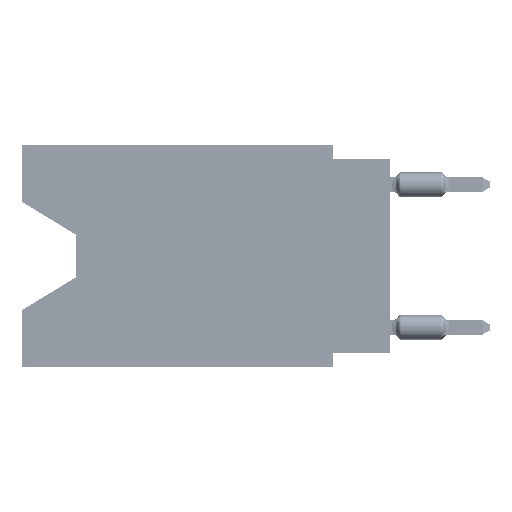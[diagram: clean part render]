
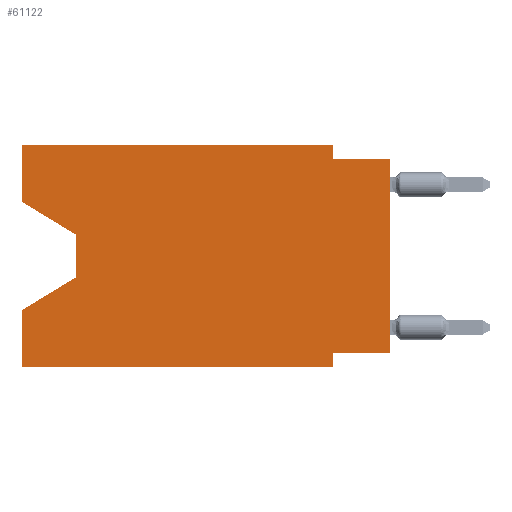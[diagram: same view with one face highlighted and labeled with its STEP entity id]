
A CAD part, left-side view. The second image highlights one B-rep face of the part: STEP entity #61122.
In plain terms, the highlighted planar face has unit normal (-1, 0, 0).
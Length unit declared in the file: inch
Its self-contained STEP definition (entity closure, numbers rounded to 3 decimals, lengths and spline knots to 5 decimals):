
#2537 = EDGE_CURVE ( 'NONE', #41093, #14408, #57321, .T. ) ;
#3447 = EDGE_CURVE ( 'NONE', #55523, #82856, #81582, .T. ) ;
#7333 = ORIENTED_EDGE ( 'NONE', *, *, #63352, .T. ) ;
#8755 = CARTESIAN_POINT ( 'NONE',  ( 0., 0.645, 0. ) ) ;
#10190 = CARTESIAN_POINT ( 'NONE',  ( 0., 0.55, -0.158 ) ) ;
#10412 = ORIENTED_EDGE ( 'NONE', *, *, #85888, .T. ) ;
#11463 = VECTOR ( 'NONE', #12196, 39.37008 ) ;
#11960 = VECTOR ( 'NONE', #19032, 39.37008 ) ;
#12196 = DIRECTION ( 'NONE',  ( 0., -1., 0. ) ) ;
#12523 = PLANE ( 'NONE',  #64655 ) ;
#13416 = EDGE_CURVE ( 'NONE', #74744, #78034, #83284, .T. ) ;
#14408 = VERTEX_POINT ( 'NONE', #86956 ) ;
#14609 = LINE ( 'NONE', #68600, #82250 ) ;
#16934 = CARTESIAN_POINT ( 'NONE',  ( 0., 0.645, 0. ) ) ;
#17168 = ORIENTED_EDGE ( 'NONE', *, *, #3447, .T. ) ;
#19032 = DIRECTION ( 'NONE',  ( 0., -1., 0. ) ) ;
#20188 = EDGE_CURVE ( 'NONE', #36233, #23892, #87376, .T. ) ;
#20350 = ORIENTED_EDGE ( 'NONE', *, *, #71336, .F. ) ;
#20557 = ORIENTED_EDGE ( 'NONE', *, *, #60749, .F. ) ;
#21324 = EDGE_CURVE ( 'NONE', #74744, #24150, #63270, .T. ) ;
#22007 = DIRECTION ( 'NONE',  ( 0., 1., 0. ) ) ;
#22513 = CARTESIAN_POINT ( 'NONE',  ( 0., 0.1, 0. ) ) ;
#23170 = VECTOR ( 'NONE', #27937, 39.37008 ) ;
#23574 = VERTEX_POINT ( 'NONE', #49384 ) ;
#23892 = VERTEX_POINT ( 'NONE', #35782 ) ;
#24150 = VERTEX_POINT ( 'NONE', #32593 ) ;
#25736 = VERTEX_POINT ( 'NONE', #53610 ) ;
#26020 = DIRECTION ( 'NONE',  ( 1., 0., 0. ) ) ;
#27937 = DIRECTION ( 'NONE',  ( 0., 0., -1. ) ) ;
#28050 = CARTESIAN_POINT ( 'NONE',  ( 0., 0.1, -0.39 ) ) ;
#28785 = LINE ( 'NONE', #56192, #43084 ) ;
#29434 = EDGE_CURVE ( 'NONE', #41093, #55523, #59913, .T. ) ;
#32593 = CARTESIAN_POINT ( 'NONE',  ( 0., 0.645, -0.28975 ) ) ;
#32743 = LINE ( 'NONE', #60601, #38855 ) ;
#34798 = CARTESIAN_POINT ( 'NONE',  ( 0., 0.645, -0.10025 ) ) ;
#35300 = DIRECTION ( 'NONE',  ( 0., 0.855, -0.519 ) ) ;
#35782 = CARTESIAN_POINT ( 'NONE',  ( 0., 0., -0.025 ) ) ;
#36233 = VERTEX_POINT ( 'NONE', #56126 ) ;
#38855 = VECTOR ( 'NONE', #88475, 39.37008 ) ;
#39813 = CARTESIAN_POINT ( 'NONE',  ( 0., 0.55, -0.158 ) ) ;
#40796 = VECTOR ( 'NONE', #67232, 39.37008 ) ;
#41093 = VERTEX_POINT ( 'NONE', #34798 ) ;
#43084 = VECTOR ( 'NONE', #59317, 39.37008 ) ;
#44087 = EDGE_CURVE ( 'NONE', #67580, #36233, #63007, .T. ) ;
#46697 = DIRECTION ( 'NONE',  ( 0., 0., -1. ) ) ;
#47963 = VECTOR ( 'NONE', #22007, 39.37008 ) ;
#49384 = CARTESIAN_POINT ( 'NONE',  ( 0., 0.1, -0.365 ) ) ;
#53610 = CARTESIAN_POINT ( 'NONE',  ( 0., 0., -0.365 ) ) ;
#55304 = ORIENTED_EDGE ( 'NONE', *, *, #20188, .F. ) ;
#55388 = ORIENTED_EDGE ( 'NONE', *, *, #60904, .F. ) ;
#55523 = VERTEX_POINT ( 'NONE', #10190 ) ;
#56126 = CARTESIAN_POINT ( 'NONE',  ( 0., 0.1, -0.025 ) ) ;
#56192 = CARTESIAN_POINT ( 'NONE',  ( 0., 0.1, -0.39 ) ) ;
#56415 = DIRECTION ( 'NONE',  ( 0., 0., 1. ) ) ;
#57321 = LINE ( 'NONE', #8755, #66906 ) ;
#59317 = DIRECTION ( 'NONE',  ( 0., 0., -1. ) ) ;
#59913 = LINE ( 'NONE', #74269, #81090 ) ;
#60601 = CARTESIAN_POINT ( 'NONE',  ( 0., 0., 0. ) ) ;
#60749 = EDGE_CURVE ( 'NONE', #14408, #67580, #73793, .T. ) ;
#60904 = EDGE_CURVE ( 'NONE', #23574, #78034, #28785, .T. ) ;
#61122 = ADVANCED_FACE ( 'NONE', ( #66949 ), #12523, .F. ) ;
#63007 = LINE ( 'NONE', #22513, #23170 ) ;
#63072 = DIRECTION ( 'NONE',  ( 0., -1., 0. ) ) ;
#63270 = LINE ( 'NONE', #16934, #69340 ) ;
#63352 = EDGE_CURVE ( 'NONE', #25736, #23892, #32743, .T. ) ;
#64655 = AXIS2_PLACEMENT_3D ( 'NONE', #87613, #26020, #46697 ) ;
#65854 = CARTESIAN_POINT ( 'NONE',  ( 0., 0.645, -0.39 ) ) ;
#66906 = VECTOR ( 'NONE', #56415, 39.37008 ) ;
#66949 = FACE_OUTER_BOUND ( 'NONE', #77417, .T. ) ;
#67232 = DIRECTION ( 'NONE',  ( 0., 0., -1. ) ) ;
#67580 = VERTEX_POINT ( 'NONE', #83609 ) ;
#68066 = ORIENTED_EDGE ( 'NONE', *, *, #2537, .F. ) ;
#68600 = CARTESIAN_POINT ( 'NONE',  ( 0., 0.55, -0.232 ) ) ;
#69019 = ORIENTED_EDGE ( 'NONE', *, *, #21324, .F. ) ;
#69340 = VECTOR ( 'NONE', #71774, 39.37008 ) ;
#71006 = LINE ( 'NONE', #78178, #47963 ) ;
#71336 = EDGE_CURVE ( 'NONE', #25736, #23574, #71006, .T. ) ;
#71774 = DIRECTION ( 'NONE',  ( 0., 0., 1. ) ) ;
#72477 = ORIENTED_EDGE ( 'NONE', *, *, #29434, .T. ) ;
#73793 = LINE ( 'NONE', #75105, #11463 ) ;
#74269 = CARTESIAN_POINT ( 'NONE',  ( 0., 0.645, -0.10025 ) ) ;
#74744 = VERTEX_POINT ( 'NONE', #65854 ) ;
#75105 = CARTESIAN_POINT ( 'NONE',  ( 0., 0.645, 0. ) ) ;
#75768 = ORIENTED_EDGE ( 'NONE', *, *, #13416, .T. ) ;
#77291 = CARTESIAN_POINT ( 'NONE',  ( 0., 0.55, -0.232 ) ) ;
#77417 = EDGE_LOOP ( 'NONE', ( #72477, #17168, #10412, #69019, #75768, #55388, #20350, #7333, #55304, #78221, #20557, #68066 ) ) ;
#78034 = VERTEX_POINT ( 'NONE', #28050 ) ;
#78178 = CARTESIAN_POINT ( 'NONE',  ( 0., 0., -0.365 ) ) ;
#78221 = ORIENTED_EDGE ( 'NONE', *, *, #44087, .F. ) ;
#80606 = CARTESIAN_POINT ( 'NONE',  ( 0., 0., -0.025 ) ) ;
#81090 = VECTOR ( 'NONE', #81885, 39.37008 ) ;
#81582 = LINE ( 'NONE', #39813, #40796 ) ;
#81885 = DIRECTION ( 'NONE',  ( 0., -0.855, -0.519 ) ) ;
#82250 = VECTOR ( 'NONE', #35300, 39.37008 ) ;
#82856 = VERTEX_POINT ( 'NONE', #77291 ) ;
#83016 = VECTOR ( 'NONE', #63072, 39.37008 ) ;
#83284 = LINE ( 'NONE', #88707, #83016 ) ;
#83609 = CARTESIAN_POINT ( 'NONE',  ( 0., 0.1, 0. ) ) ;
#85888 = EDGE_CURVE ( 'NONE', #82856, #24150, #14609, .T. ) ;
#86956 = CARTESIAN_POINT ( 'NONE',  ( 0., 0.645, 0. ) ) ;
#87376 = LINE ( 'NONE', #80606, #11960 ) ;
#87613 = CARTESIAN_POINT ( 'NONE',  ( 0., 0.645, 0. ) ) ;
#88475 = DIRECTION ( 'NONE',  ( 0., 0., 1. ) ) ;
#88707 = CARTESIAN_POINT ( 'NONE',  ( 0., 0.645, -0.39 ) ) ;
